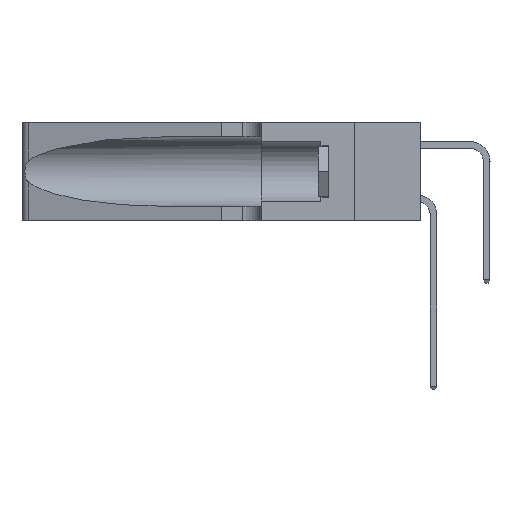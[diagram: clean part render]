
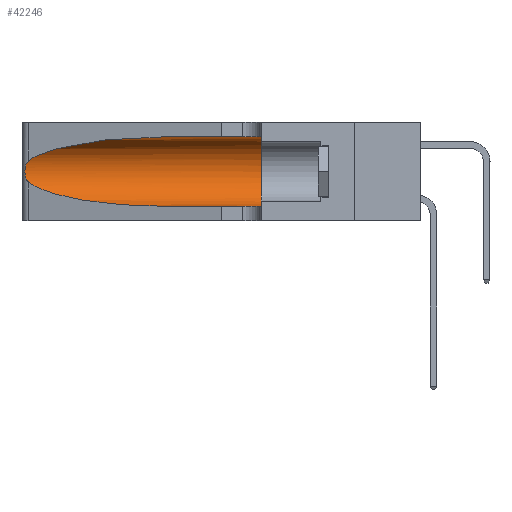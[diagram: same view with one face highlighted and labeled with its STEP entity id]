
A CAD part, left-side view. The second image highlights one B-rep face of the part: STEP entity #42246.
In plain terms, the highlighted cylindrical face has radius 3.308 mm (diameter 6.617 mm), a partial arc.
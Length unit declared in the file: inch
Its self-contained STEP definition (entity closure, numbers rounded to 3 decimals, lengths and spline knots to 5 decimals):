
#1724 = CARTESIAN_POINT ( 'NONE',  ( 0.26017, 1.23833, 0.17102 ) ) ;
#1790 = LINE ( 'NONE', #43194, #16482 ) ;
#3008 = AXIS2_PLACEMENT_3D ( 'NONE', #18609, #41976, #16234 ) ;
#4343 = CARTESIAN_POINT ( 'NONE',  ( 0.25487, 1.22718, 0.22369 ) ) ;
#4505 = ORIENTED_EDGE ( 'NONE', *, *, #11767, .T. ) ;
#4565 = ORIENTED_EDGE ( 'NONE', *, *, #20076, .T. ) ;
#6823 = CARTESIAN_POINT ( 'NONE',  ( 0.25487, 1.22718, 0.22369 ) ) ;
#7011 = CARTESIAN_POINT ( 'NONE',  ( 0.1305, 0.72297, 0.31525 ) ) ;
#7265 = CARTESIAN_POINT ( 'NONE',  ( 0.26018, 1.23835, 0.19895 ) ) ;
#7388 = EDGE_CURVE ( 'NONE', #40062, #16557, #19941, .T. ) ;
#7816 = DIRECTION ( 'NONE',  ( 0., 0., -1. ) ) ;
#8477 =( BOUNDED_CURVE ( )  B_SPLINE_CURVE ( 3, ( #15378, #41856, #22125, #18887 ),
 .UNSPECIFIED., .F., .F. ) 
 B_SPLINE_CURVE_WITH_KNOTS ( ( 4, 4 ),
 ( 3.44316, 4.71239 ),
 .UNSPECIFIED. ) 
 CURVE ( )  GEOMETRIC_REPRESENTATION_ITEM ( )  RATIONAL_B_SPLINE_CURVE ( ( 1., 0.87, 0.87, 1. ) ) 
 REPRESENTATION_ITEM ( '' )  );
#8788 = CARTESIAN_POINT ( 'NONE',  ( 0.18966, 0.96281, 0.31525 ) ) ;
#10315 = AXIS2_PLACEMENT_3D ( 'NONE', #31687, #41032, #7816 ) ;
#10995 = CARTESIAN_POINT ( 'NONE',  ( 0.25487, 1.22718, 0.14631 ) ) ;
#11071 = CARTESIAN_POINT ( 'NONE',  ( 0.26075, 1.23896, 0.178 ) ) ;
#11524 = DIRECTION ( 'NONE',  ( 0., -1., 0. ) ) ;
#11767 = EDGE_CURVE ( 'NONE', #17390, #30049, #26193, .T. ) ;
#12135 = CARTESIAN_POINT ( 'NONE',  ( 0.2373, 1.15595, 0.28018 ) ) ;
#13052 = CARTESIAN_POINT ( 'NONE',  ( 0.25487, 1.22718, 0.22369 ) ) ;
#13602 = CARTESIAN_POINT ( 'NONE',  ( 0.25787, 1.23484, 0.2124 ) ) ;
#13640 = CARTESIAN_POINT ( 'NONE',  ( 0.1305, 0.35, 0.05475 ) ) ;
#15155 = CARTESIAN_POINT ( 'NONE',  ( 0.1305, 0.72297, 0.05475 ) ) ;
#15324 = ORIENTED_EDGE ( 'NONE', *, *, #21205, .F. ) ;
#15378 = CARTESIAN_POINT ( 'NONE',  ( 0.25487, 1.22718, 0.14631 ) ) ;
#15394 = CARTESIAN_POINT ( 'NONE',  ( 0.1305, 0.72297, 0.31525 ) ) ;
#16234 = DIRECTION ( 'NONE',  ( 0., 0., 1. ) ) ;
#16482 = VECTOR ( 'NONE', #11524, 39.37008 ) ;
#16557 = VERTEX_POINT ( 'NONE', #13640 ) ;
#16634 = CARTESIAN_POINT ( 'NONE',  ( 0.1305, 1.61858, 0.05475 ) ) ;
#16855 = CARTESIAN_POINT ( 'NONE',  ( 0.26075, 1.23896, 0.19203 ) ) ;
#17390 = VERTEX_POINT ( 'NONE', #4343 ) ;
#18264 = FACE_OUTER_BOUND ( 'NONE', #35595, .T. ) ;
#18609 = CARTESIAN_POINT ( 'NONE',  ( 0.1305, 0.35, 0.185 ) ) ;
#18887 = CARTESIAN_POINT ( 'NONE',  ( 0.1305, 0.72297, 0.05475 ) ) ;
#19866 = VERTEX_POINT ( 'NONE', #25993 ) ;
#19941 = LINE ( 'NONE', #16634, #41933 ) ;
#20076 = EDGE_CURVE ( 'NONE', #30049, #40062, #8477, .T. ) ;
#20502 = CARTESIAN_POINT ( 'NONE',  ( 0.25487, 1.22718, 0.14631 ) ) ;
#21205 = EDGE_CURVE ( 'NONE', #19866, #16557, #36072, .T. ) ;
#22125 = CARTESIAN_POINT ( 'NONE',  ( 0.18966, 0.96281, 0.05475 ) ) ;
#23991 = CARTESIAN_POINT ( 'NONE',  ( 0.25854, 1.2359, 0.20912 ) ) ;
#24229 = EDGE_CURVE ( 'NONE', #35077, #19866, #1790, .T. ) ;
#25572 = ORIENTED_EDGE ( 'NONE', *, *, #24229, .F. ) ;
#25993 = CARTESIAN_POINT ( 'NONE',  ( 0.1305, 0.35, 0.31525 ) ) ;
#26094 = CARTESIAN_POINT ( 'NONE',  ( 0.25555, 1.22994, 0.2215 ) ) ;
#26188 = CARTESIAN_POINT ( 'NONE',  ( 0.25856, 1.23593, 0.16098 ) ) ;
#26193 = B_SPLINE_CURVE_WITH_KNOTS ( 'NONE', 3,
 ( #13052, #26094, #29542, #13602, #23991, #7265, #16855, #11071, #1724, #26188, #33682, #40816, #27794, #20502 ),
 .UNSPECIFIED., .F., .F.,
 ( 4, 2, 2, 2, 2, 2, 4 ),
 ( 0., 0.00027, 0.00053, 0.00107, 0.0016, 0.00187, 0.00214 ),
 .UNSPECIFIED. ) ;
#26709 =( BOUNDED_CURVE ( )  B_SPLINE_CURVE ( 3, ( #15394, #8788, #12135, #6823 ),
 .UNSPECIFIED., .F., .F. ) 
 B_SPLINE_CURVE_WITH_KNOTS ( ( 4, 4 ),
 ( 1.5708, 2.84003 ),
 .UNSPECIFIED. ) 
 CURVE ( )  GEOMETRIC_REPRESENTATION_ITEM ( )  RATIONAL_B_SPLINE_CURVE ( ( 1., 0.87, 0.87, 1. ) ) 
 REPRESENTATION_ITEM ( '' )  );
#27794 = CARTESIAN_POINT ( 'NONE',  ( 0.25555, 1.22993, 0.14849 ) ) ;
#28376 = EDGE_CURVE ( 'NONE', #35077, #17390, #26709, .T. ) ;
#29542 = CARTESIAN_POINT ( 'NONE',  ( 0.25639, 1.23184, 0.21858 ) ) ;
#30049 = VERTEX_POINT ( 'NONE', #10995 ) ;
#31687 = CARTESIAN_POINT ( 'NONE',  ( 0.1305, 1.61858, 0.185 ) ) ;
#33682 = CARTESIAN_POINT ( 'NONE',  ( 0.25789, 1.23486, 0.15765 ) ) ;
#35077 = VERTEX_POINT ( 'NONE', #7011 ) ;
#35595 = EDGE_LOOP ( 'NONE', ( #41585, #4505, #4565, #37820, #15324, #25572 ) ) ;
#36072 = CIRCLE ( 'NONE', #3008, 0.13025 ) ;
#37820 = ORIENTED_EDGE ( 'NONE', *, *, #7388, .T. ) ;
#39707 = DIRECTION ( 'NONE',  ( 0., -1., 0. ) ) ;
#40062 = VERTEX_POINT ( 'NONE', #15155 ) ;
#40816 = CARTESIAN_POINT ( 'NONE',  ( 0.25639, 1.23186, 0.15144 ) ) ;
#41032 = DIRECTION ( 'NONE',  ( 0., -1., 0. ) ) ;
#41585 = ORIENTED_EDGE ( 'NONE', *, *, #28376, .T. ) ;
#41787 = CYLINDRICAL_SURFACE ( 'NONE', #10315, 0.13025 ) ;
#41856 = CARTESIAN_POINT ( 'NONE',  ( 0.2373, 1.15595, 0.08982 ) ) ;
#41933 = VECTOR ( 'NONE', #39707, 39.37008 ) ;
#41976 = DIRECTION ( 'NONE',  ( 0., 1., 0. ) ) ;
#42246 = ADVANCED_FACE ( 'NONE', ( #18264 ), #41787, .F. ) ;
#43194 = CARTESIAN_POINT ( 'NONE',  ( 0.1305, 1.61858, 0.31525 ) ) ;
